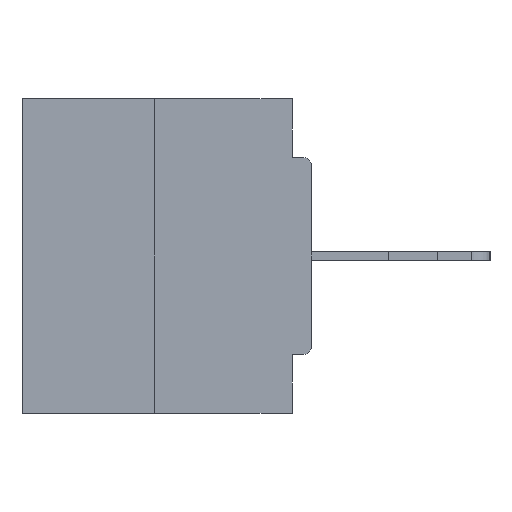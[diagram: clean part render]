
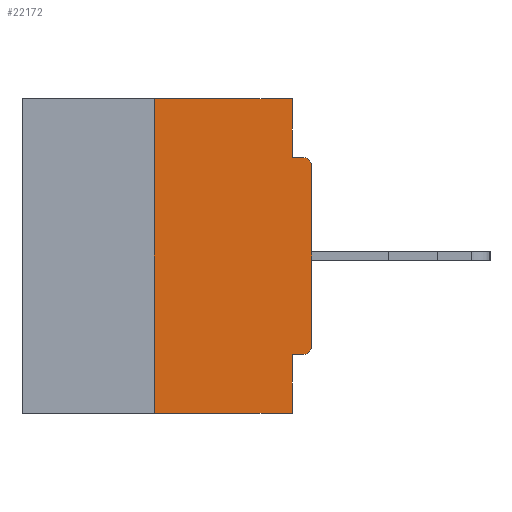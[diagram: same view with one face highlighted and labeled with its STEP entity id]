
A CAD part, left-side view. The second image highlights one B-rep face of the part: STEP entity #22172.
In plain terms, the highlighted planar face has unit normal (-1, 0, 0).
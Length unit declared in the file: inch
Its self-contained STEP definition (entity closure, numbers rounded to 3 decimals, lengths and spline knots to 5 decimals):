
#1206 = ORIENTED_EDGE ( 'NONE', *, *, #21241, .F. ) ;
#1508 = VECTOR ( 'NONE', #25147, 39.37008 ) ;
#1822 = CARTESIAN_POINT ( 'NONE',  ( 0., 0.46, -0.5 ) ) ;
#1828 = DIRECTION ( 'NONE',  ( 0., -1., 0. ) ) ;
#2433 = EDGE_CURVE ( 'NONE', #18381, #8448, #25047, .T. ) ;
#2553 = LINE ( 'NONE', #12037, #15277 ) ;
#3512 = EDGE_CURVE ( 'NONE', #16035, #26121, #23509, .T. ) ;
#3901 = DIRECTION ( 'NONE',  ( 0., 0., -1. ) ) ;
#4478 = LINE ( 'NONE', #30454, #6909 ) ;
#4548 = CARTESIAN_POINT ( 'NONE',  ( 0., 0.031, -0.4065 ) ) ;
#4642 = EDGE_CURVE ( 'NONE', #16035, #27920, #8348, .T. ) ;
#5701 = AXIS2_PLACEMENT_3D ( 'NONE', #20229, #29121, #22746 ) ;
#6119 = CARTESIAN_POINT ( 'NONE',  ( 0., 0.015, -0.1085 ) ) ;
#6204 = ORIENTED_EDGE ( 'NONE', *, *, #9382, .T. ) ;
#6716 = EDGE_CURVE ( 'NONE', #23784, #26121, #4478, .T. ) ;
#6909 = VECTOR ( 'NONE', #13684, 39.37008 ) ;
#7182 = EDGE_LOOP ( 'NONE', ( #1206, #18900, #16960, #10616, #18886, #27334, #6204, #18223, #8150, #22829 ) ) ;
#7436 = EDGE_CURVE ( 'NONE', #24602, #28298, #19564, .T. ) ;
#7704 = VECTOR ( 'NONE', #1828, 39.37008 ) ;
#8150 = ORIENTED_EDGE ( 'NONE', *, *, #20727, .F. ) ;
#8199 = CARTESIAN_POINT ( 'NONE',  ( 0., 0., -0.1085 ) ) ;
#8209 = CARTESIAN_POINT ( 'NONE',  ( 0., 0.015, -0.3915 ) ) ;
#8348 = LINE ( 'NONE', #15946, #1508 ) ;
#8448 = VERTEX_POINT ( 'NONE', #20636 ) ;
#8726 = CARTESIAN_POINT ( 'NONE',  ( 0., 0.015, -0.0935 ) ) ;
#8772 = CARTESIAN_POINT ( 'NONE',  ( 0., 0., -0.4065 ) ) ;
#9382 = EDGE_CURVE ( 'NONE', #28298, #23642, #24441, .T. ) ;
#9472 = VERTEX_POINT ( 'NONE', #8726 ) ;
#9802 = DIRECTION ( 'NONE',  ( 0., -1., 0. ) ) ;
#10357 = VECTOR ( 'NONE', #27129, 39.37008 ) ;
#10616 = ORIENTED_EDGE ( 'NONE', *, *, #6716, .F. ) ;
#11572 = EDGE_CURVE ( 'NONE', #23642, #9472, #29605, .T. ) ;
#11780 = CARTESIAN_POINT ( 'NONE',  ( 0., 0.46, 0. ) ) ;
#12011 = CARTESIAN_POINT ( 'NONE',  ( 0., 0.031, -0.5 ) ) ;
#12037 = CARTESIAN_POINT ( 'NONE',  ( 0., 0., -0.0935 ) ) ;
#13684 = DIRECTION ( 'NONE',  ( 0., 0., -1. ) ) ;
#14021 = LINE ( 'NONE', #8772, #24276 ) ;
#14078 = VECTOR ( 'NONE', #19382, 39.37008 ) ;
#14259 = CARTESIAN_POINT ( 'NONE',  ( 0., 0.015, -0.4065 ) ) ;
#14440 = AXIS2_PLACEMENT_3D ( 'NONE', #6119, #24981, #18028 ) ;
#14470 = CARTESIAN_POINT ( 'NONE',  ( 0., 0., -0.3915 ) ) ;
#14724 = FACE_OUTER_BOUND ( 'NONE', #7182, .T. ) ;
#14940 = CARTESIAN_POINT ( 'NONE',  ( 0., 0., 0. ) ) ;
#15277 = VECTOR ( 'NONE', #9802, 39.37008 ) ;
#15311 = PLANE ( 'NONE',  #5701 ) ;
#15946 = CARTESIAN_POINT ( 'NONE',  ( 0., 0.25, 0. ) ) ;
#16035 = VERTEX_POINT ( 'NONE', #19830 ) ;
#16960 = ORIENTED_EDGE ( 'NONE', *, *, #3512, .T. ) ;
#18028 = DIRECTION ( 'NONE',  ( 0., 0., -1. ) ) ;
#18223 = ORIENTED_EDGE ( 'NONE', *, *, #11572, .T. ) ;
#18381 = VERTEX_POINT ( 'NONE', #18763 ) ;
#18390 = EDGE_CURVE ( 'NONE', #24602, #23784, #14021, .T. ) ;
#18753 = DIRECTION ( 'NONE',  ( 0., -1., 0. ) ) ;
#18763 = CARTESIAN_POINT ( 'NONE',  ( 0., 0.031, 0. ) ) ;
#18886 = ORIENTED_EDGE ( 'NONE', *, *, #18390, .F. ) ;
#18900 = ORIENTED_EDGE ( 'NONE', *, *, #4642, .F. ) ;
#19382 = DIRECTION ( 'NONE',  ( 0., 0., 1. ) ) ;
#19564 = CIRCLE ( 'NONE', #26105, 0.015 ) ;
#19749 = CARTESIAN_POINT ( 'NONE',  ( 0., 0.25, 0. ) ) ;
#19830 = CARTESIAN_POINT ( 'NONE',  ( 0., 0.25, -0.5 ) ) ;
#20229 = CARTESIAN_POINT ( 'NONE',  ( 0., 0.46, 0. ) ) ;
#20636 = CARTESIAN_POINT ( 'NONE',  ( 0., 0.031, -0.0935 ) ) ;
#20727 = EDGE_CURVE ( 'NONE', #8448, #9472, #2553, .T. ) ;
#21241 = EDGE_CURVE ( 'NONE', #27920, #18381, #26365, .T. ) ;
#22172 = ADVANCED_FACE ( 'NONE', ( #14724 ), #15311, .F. ) ;
#22746 = DIRECTION ( 'NONE',  ( 0., 0., -1. ) ) ;
#22829 = ORIENTED_EDGE ( 'NONE', *, *, #2433, .F. ) ;
#23509 = LINE ( 'NONE', #1822, #24701 ) ;
#23642 = VERTEX_POINT ( 'NONE', #8199 ) ;
#23784 = VERTEX_POINT ( 'NONE', #4548 ) ;
#24276 = VECTOR ( 'NONE', #26209, 39.37008 ) ;
#24441 = LINE ( 'NONE', #14940, #14078 ) ;
#24602 = VERTEX_POINT ( 'NONE', #14259 ) ;
#24701 = VECTOR ( 'NONE', #18753, 39.37008 ) ;
#24981 = DIRECTION ( 'NONE',  ( -1., 0., 0. ) ) ;
#25047 = LINE ( 'NONE', #27587, #10357 ) ;
#25147 = DIRECTION ( 'NONE',  ( 0., 0., 1. ) ) ;
#26105 = AXIS2_PLACEMENT_3D ( 'NONE', #8209, #29445, #3901 ) ;
#26121 = VERTEX_POINT ( 'NONE', #12011 ) ;
#26209 = DIRECTION ( 'NONE',  ( 0., 1., 0. ) ) ;
#26365 = LINE ( 'NONE', #11780, #7704 ) ;
#27129 = DIRECTION ( 'NONE',  ( 0., 0., -1. ) ) ;
#27334 = ORIENTED_EDGE ( 'NONE', *, *, #7436, .T. ) ;
#27587 = CARTESIAN_POINT ( 'NONE',  ( 0., 0.031, 0. ) ) ;
#27920 = VERTEX_POINT ( 'NONE', #19749 ) ;
#28298 = VERTEX_POINT ( 'NONE', #14470 ) ;
#29121 = DIRECTION ( 'NONE',  ( 1., 0., 0. ) ) ;
#29445 = DIRECTION ( 'NONE',  ( -1., 0., 0. ) ) ;
#29605 = CIRCLE ( 'NONE', #14440, 0.015 ) ;
#30454 = CARTESIAN_POINT ( 'NONE',  ( 0., 0.031, -0.5 ) ) ;
